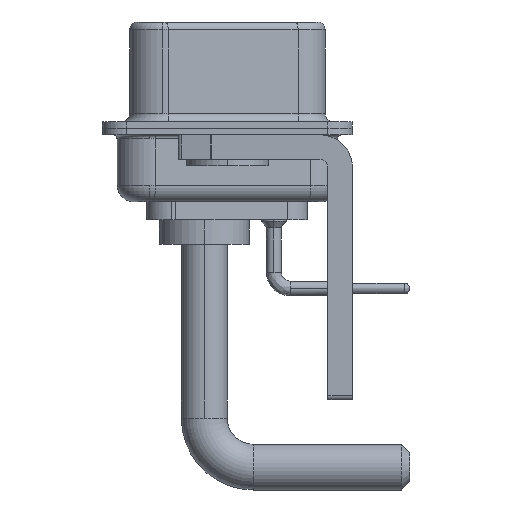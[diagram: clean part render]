
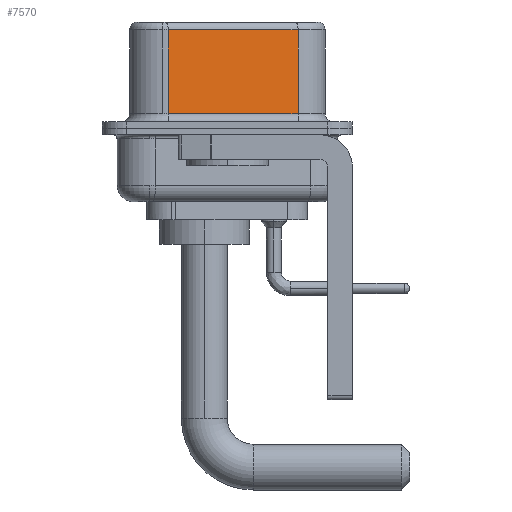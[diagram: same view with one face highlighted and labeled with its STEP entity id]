
A CAD part, left-side view. The second image highlights one B-rep face of the part: STEP entity #7570.
In plain terms, the highlighted planar face has unit normal (-0.985, -0.174, 0).
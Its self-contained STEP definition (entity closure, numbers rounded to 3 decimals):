
#697 = LINE ( 'NONE', #10214, #15483 ) ;
#759 = LINE ( 'NONE', #12254, #1725 ) ;
#1158 = EDGE_CURVE ( 'NONE', #21570, #20679, #759, .T. ) ;
#1639 = ORIENTED_EDGE ( 'NONE', *, *, #1158, .T. ) ;
#1725 = VECTOR ( 'NONE', #4539, 1000. ) ;
#1834 = ORIENTED_EDGE ( 'NONE', *, *, #17805, .T. ) ;
#1854 = ORIENTED_EDGE ( 'NONE', *, *, #9113, .T. ) ;
#3356 = DIRECTION ( 'NONE',  ( 0., 0., -1. ) ) ;
#4515 = DIRECTION ( 'NONE',  ( -0.174, 0.985, 0. ) ) ;
#4539 = DIRECTION ( 'NONE',  ( -0.174, 0.985, 0. ) ) ;
#6459 = VERTEX_POINT ( 'NONE', #23173 ) ;
#7365 = CARTESIAN_POINT ( 'NONE',  ( 3.73, 3.628, 6.52 ) ) ;
#7570 = ADVANCED_FACE ( 'NONE', ( #8508 ), #8369, .F. ) ;
#8369 = PLANE ( 'NONE',  #20430 ) ;
#8508 = FACE_OUTER_BOUND ( 'NONE', #24121, .T. ) ;
#8879 = ORIENTED_EDGE ( 'NONE', *, *, #10823, .F. ) ;
#9113 = EDGE_CURVE ( 'NONE', #20679, #10962, #16821, .T. ) ;
#10214 = CARTESIAN_POINT ( 'NONE',  ( 5.132, -4.322, 0.9 ) ) ;
#10823 = EDGE_CURVE ( 'NONE', #21570, #6459, #16918, .T. ) ;
#10962 = VERTEX_POINT ( 'NONE', #22552 ) ;
#11216 = CARTESIAN_POINT ( 'NONE',  ( 5.132, -4.322, 6.52 ) ) ;
#11829 = DIRECTION ( 'NONE',  ( 0.174, -0.985, 0. ) ) ;
#12254 = CARTESIAN_POINT ( 'NONE',  ( 5.132, -4.322, 6.02 ) ) ;
#14946 = DIRECTION ( 'NONE',  ( 0., 0., -1. ) ) ;
#15325 = VECTOR ( 'NONE', #3356, 1000. ) ;
#15483 = VECTOR ( 'NONE', #11829, 1000. ) ;
#15829 = DIRECTION ( 'NONE',  ( 0.985, 0.174, 0. ) ) ;
#16821 = LINE ( 'NONE', #7365, #23132 ) ;
#16918 = LINE ( 'NONE', #11216, #15325 ) ;
#17805 = EDGE_CURVE ( 'NONE', #10962, #6459, #697, .T. ) ;
#20430 = AXIS2_PLACEMENT_3D ( 'NONE', #23693, #15829, #4515 ) ;
#20679 = VERTEX_POINT ( 'NONE', #22725 ) ;
#21570 = VERTEX_POINT ( 'NONE', #22454 ) ;
#22454 = CARTESIAN_POINT ( 'NONE',  ( 5.132, -4.322, 6.02 ) ) ;
#22552 = CARTESIAN_POINT ( 'NONE',  ( 3.73, 3.628, 0.9 ) ) ;
#22725 = CARTESIAN_POINT ( 'NONE',  ( 3.73, 3.628, 6.02 ) ) ;
#23132 = VECTOR ( 'NONE', #14946, 1000. ) ;
#23173 = CARTESIAN_POINT ( 'NONE',  ( 5.132, -4.322, 0.9 ) ) ;
#23693 = CARTESIAN_POINT ( 'NONE',  ( 5.132, -4.322, 6.52 ) ) ;
#24121 = EDGE_LOOP ( 'NONE', ( #8879, #1639, #1854, #1834 ) ) ;
